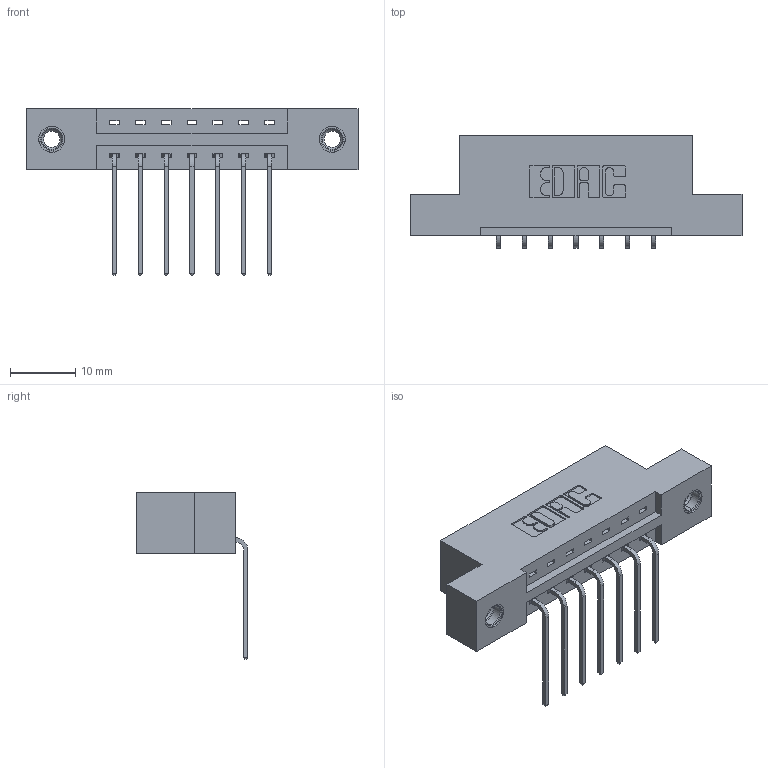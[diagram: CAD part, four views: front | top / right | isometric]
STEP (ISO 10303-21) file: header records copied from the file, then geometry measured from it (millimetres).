
FILE_DESCRIPTION (( 'STEP AP203' ), '1' );
FILE_NAME ('387-007-559-107.STEP', '2018-08-13T06:30:56', ( '' ), ( '' ), 'SwSTEP 2.0', 'SolidWorks 2016', '' );
FILE_SCHEMA (( 'CONFIG_CONTROL_DESIGN' ));
Length unit declared in the file: inch
Products named in the file (4): 337 Part_Flush Mounting Lugs - 0.156 Dia-TI; 345-292-001_558 559 Tail - 1; 345-250-001_345-250-005-103; 387-007-559-107
Assembly tree (10 placements, depth 2):
  387-007-559-107
    337 Part_Flush Mounting Lugs - 0.156 Dia-TI
    345-292-001_558 559 Tail - 1  x7
    345-250-001_345-250-005-103  x2
Bounding box: 50.75 x 17.09 x 25.53 mm (x, y, z)
Volume: 4846.3 mm3; surface area: 4998.1 mm2
Topology: 10 solids, 10 shells, 622 faces, 1805 edges, 1186 vertices
Faces by surface type: plane 438, cylinder 168, cone 12, torus 4
Entity records: 11000 total; most frequent: CARTESIAN_POINT 1894, ORIENTED_EDGE 1830, DIRECTION 1699, EDGE_CURVE 915, LINE 767, VECTOR 767, VERTEX_POINT 604, AXIS2_PLACEMENT_3D 466
